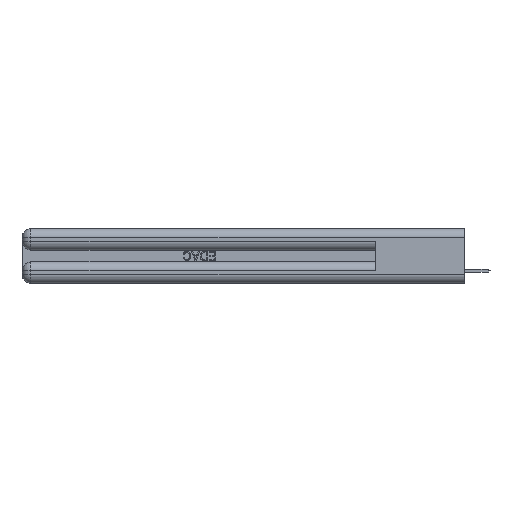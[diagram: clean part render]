
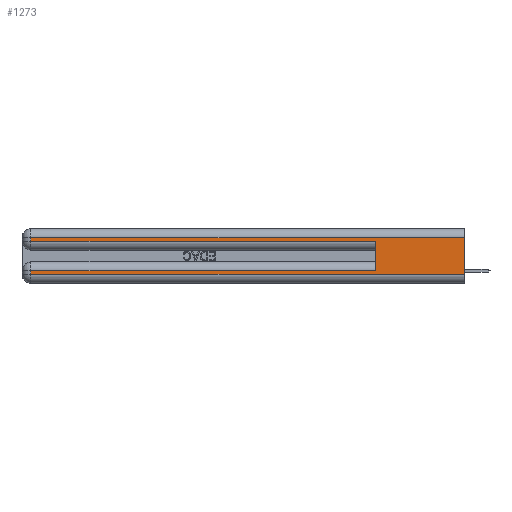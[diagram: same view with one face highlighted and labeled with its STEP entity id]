
A CAD part, left-side view. The second image highlights one B-rep face of the part: STEP entity #1273.
In plain terms, the highlighted planar face has unit normal (-1, 0, 0).
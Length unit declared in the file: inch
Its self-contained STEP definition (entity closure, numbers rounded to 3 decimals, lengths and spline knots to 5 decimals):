
#299 = EDGE_CURVE ( 'NONE', #36227, #35849, #7851, .T. ) ;
#674 = DIRECTION ( 'NONE',  ( 0., 0., -1. ) ) ;
#760 = CARTESIAN_POINT ( 'NONE',  ( 0., 2.94, 0.085 ) ) ;
#771 = LINE ( 'NONE', #26501, #31133 ) ;
#894 = VECTOR ( 'NONE', #43266, 39.37008 ) ;
#1273 = ADVANCED_FACE ( 'NONE', ( #17470 ), #13123, .F. ) ;
#1426 = CARTESIAN_POINT ( 'NONE',  ( 0., 0.6, 0.085 ) ) ;
#1466 = VERTEX_POINT ( 'NONE', #23408 ) ;
#1779 = DIRECTION ( 'NONE',  ( 1., 0., 0. ) ) ;
#2864 = DIRECTION ( 'NONE',  ( 0., 0., -1. ) ) ;
#3368 = CARTESIAN_POINT ( 'NONE',  ( 0., 2.94, 0.37 ) ) ;
#4009 = VERTEX_POINT ( 'NONE', #26970 ) ;
#4365 = VECTOR ( 'NONE', #674, 39.37008 ) ;
#7493 = ORIENTED_EDGE ( 'NONE', *, *, #52835, .T. ) ;
#7851 = LINE ( 'NONE', #38891, #14376 ) ;
#7858 = ORIENTED_EDGE ( 'NONE', *, *, #8546, .T. ) ;
#8135 = EDGE_CURVE ( 'NONE', #39660, #4009, #771, .T. ) ;
#8546 = EDGE_CURVE ( 'NONE', #49101, #36227, #23884, .T. ) ;
#9671 = ORIENTED_EDGE ( 'NONE', *, *, #32440, .T. ) ;
#10050 = CARTESIAN_POINT ( 'NONE',  ( 0., 0.6, 0.285 ) ) ;
#12737 = CARTESIAN_POINT ( 'NONE',  ( 0., 0., 0.31 ) ) ;
#13123 = PLANE ( 'NONE',  #35212 ) ;
#14376 = VECTOR ( 'NONE', #18181, 39.37008 ) ;
#14776 = LINE ( 'NONE', #20750, #894 ) ;
#17470 = FACE_OUTER_BOUND ( 'NONE', #30868, .T. ) ;
#18181 = DIRECTION ( 'NONE',  ( 0., -1., 0. ) ) ;
#20651 = DIRECTION ( 'NONE',  ( 0., 1., 0. ) ) ;
#20750 = CARTESIAN_POINT ( 'NONE',  ( 0., 0., 0.37 ) ) ;
#20869 = VECTOR ( 'NONE', #20651, 39.37008 ) ;
#21259 = ORIENTED_EDGE ( 'NONE', *, *, #41251, .T. ) ;
#21458 = EDGE_CURVE ( 'NONE', #1466, #4009, #14776, .T. ) ;
#23408 = CARTESIAN_POINT ( 'NONE',  ( 0., 0., 0.31 ) ) ;
#23884 = LINE ( 'NONE', #3368, #43730 ) ;
#24869 = DIRECTION ( 'NONE',  ( 0., 0., -1. ) ) ;
#26501 = CARTESIAN_POINT ( 'NONE',  ( 0., 0., 0.06 ) ) ;
#26970 = CARTESIAN_POINT ( 'NONE',  ( 0., 0., 0.06 ) ) ;
#28083 = ORIENTED_EDGE ( 'NONE', *, *, #21458, .F. ) ;
#30223 = DIRECTION ( 'NONE',  ( 0., 1., 0. ) ) ;
#30564 = LINE ( 'NONE', #33123, #49232 ) ;
#30614 = LINE ( 'NONE', #30699, #4365 ) ;
#30699 = CARTESIAN_POINT ( 'NONE',  ( 0., 2.94, 0.37 ) ) ;
#30868 = EDGE_LOOP ( 'NONE', ( #28083, #7493, #7858, #34803, #38449, #21259, #9671, #37515 ) ) ;
#31133 = VECTOR ( 'NONE', #43599, 39.37008 ) ;
#32128 = LINE ( 'NONE', #12737, #20869 ) ;
#32440 = EDGE_CURVE ( 'NONE', #39284, #39660, #30614, .T. ) ;
#33123 = CARTESIAN_POINT ( 'NONE',  ( 0., 0.6, 0.145 ) ) ;
#33494 = CARTESIAN_POINT ( 'NONE',  ( 0., 0., 0.37 ) ) ;
#33725 = EDGE_CURVE ( 'NONE', #37194, #35849, #30564, .T. ) ;
#34803 = ORIENTED_EDGE ( 'NONE', *, *, #299, .T. ) ;
#35174 = CARTESIAN_POINT ( 'NONE',  ( 0., 2.94, 0.31 ) ) ;
#35212 = AXIS2_PLACEMENT_3D ( 'NONE', #33494, #1779, #2864 ) ;
#35849 = VERTEX_POINT ( 'NONE', #10050 ) ;
#36227 = VERTEX_POINT ( 'NONE', #54683 ) ;
#37194 = VERTEX_POINT ( 'NONE', #1426 ) ;
#37515 = ORIENTED_EDGE ( 'NONE', *, *, #8135, .T. ) ;
#38065 = CARTESIAN_POINT ( 'NONE',  ( 0., 0., 0.085 ) ) ;
#38449 = ORIENTED_EDGE ( 'NONE', *, *, #33725, .F. ) ;
#38891 = CARTESIAN_POINT ( 'NONE',  ( 0., 0., 0.285 ) ) ;
#39284 = VERTEX_POINT ( 'NONE', #760 ) ;
#39660 = VERTEX_POINT ( 'NONE', #49568 ) ;
#41251 = EDGE_CURVE ( 'NONE', #37194, #39284, #53555, .T. ) ;
#43266 = DIRECTION ( 'NONE',  ( 0., 0., -1. ) ) ;
#43599 = DIRECTION ( 'NONE',  ( 0., -1., 0. ) ) ;
#43730 = VECTOR ( 'NONE', #24869, 39.37008 ) ;
#47690 = DIRECTION ( 'NONE',  ( 0., 0., 1. ) ) ;
#49101 = VERTEX_POINT ( 'NONE', #35174 ) ;
#49232 = VECTOR ( 'NONE', #47690, 39.37008 ) ;
#49568 = CARTESIAN_POINT ( 'NONE',  ( 0., 2.94, 0.06 ) ) ;
#52835 = EDGE_CURVE ( 'NONE', #1466, #49101, #32128, .T. ) ;
#52863 = VECTOR ( 'NONE', #30223, 39.37008 ) ;
#53555 = LINE ( 'NONE', #38065, #52863 ) ;
#54683 = CARTESIAN_POINT ( 'NONE',  ( 0., 2.94, 0.285 ) ) ;
